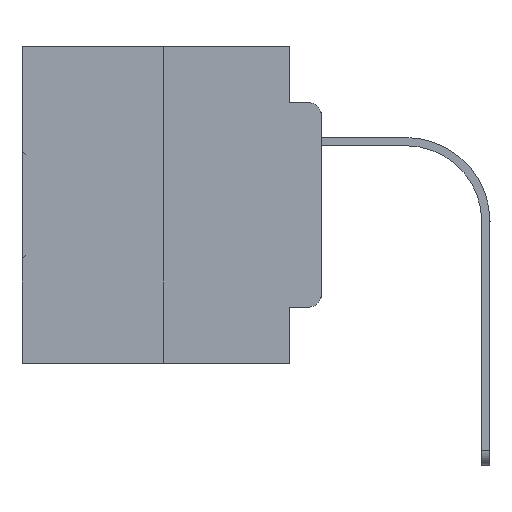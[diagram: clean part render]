
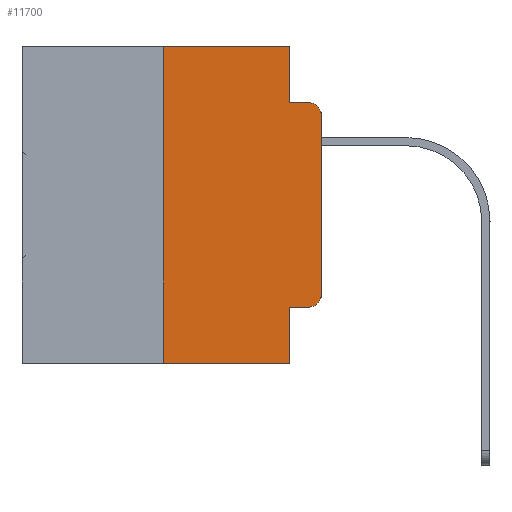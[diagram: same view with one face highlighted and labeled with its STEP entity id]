
A CAD part, left-side view. The second image highlights one B-rep face of the part: STEP entity #11700.
In plain terms, the highlighted planar face has unit normal (-1, 0, 0).
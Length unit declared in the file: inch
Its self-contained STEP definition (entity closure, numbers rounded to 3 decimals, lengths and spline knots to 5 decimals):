
#168 = DIRECTION ( 'NONE',  ( 0., 0., -1. ) ) ;
#213 = VERTEX_POINT ( 'NONE', #25439 ) ;
#641 = CARTESIAN_POINT ( 'NONE',  ( 0., 0.051, -0.5 ) ) ;
#700 = VERTEX_POINT ( 'NONE', #30990 ) ;
#843 = VERTEX_POINT ( 'NONE', #4850 ) ;
#1678 = AXIS2_PLACEMENT_3D ( 'NONE', #29289, #9576, #21879 ) ;
#1745 = DIRECTION ( 'NONE',  ( 0., -1., 0. ) ) ;
#2567 = CARTESIAN_POINT ( 'NONE',  ( 0., 0.473, 0. ) ) ;
#2694 = CIRCLE ( 'NONE', #1678, 0.02 ) ;
#2967 = DIRECTION ( 'NONE',  ( 0., 0., 1. ) ) ;
#3023 = ORIENTED_EDGE ( 'NONE', *, *, #15498, .T. ) ;
#3044 = AXIS2_PLACEMENT_3D ( 'NONE', #2567, #4975, #14767 ) ;
#3327 = CARTESIAN_POINT ( 'NONE',  ( 0., 0.051, 0. ) ) ;
#3491 = CARTESIAN_POINT ( 'NONE',  ( 0., 0.051, 0. ) ) ;
#3603 = CARTESIAN_POINT ( 'NONE',  ( 0., 0.051, -0.4115 ) ) ;
#4026 = DIRECTION ( 'NONE',  ( 0., -1., 0. ) ) ;
#4403 = VECTOR ( 'NONE', #26647, 39.37008 ) ;
#4667 = CARTESIAN_POINT ( 'NONE',  ( 0., 0.473, -0.5 ) ) ;
#4699 = LINE ( 'NONE', #7105, #4403 ) ;
#4794 = LINE ( 'NONE', #7355, #26368 ) ;
#4845 = ORIENTED_EDGE ( 'NONE', *, *, #5979, .F. ) ;
#4850 = CARTESIAN_POINT ( 'NONE',  ( 0., 0., -0.3915 ) ) ;
#4957 = VECTOR ( 'NONE', #4026, 39.37008 ) ;
#4975 = DIRECTION ( 'NONE',  ( 1., 0., 0. ) ) ;
#5979 = EDGE_CURVE ( 'NONE', #22301, #213, #17883, .T. ) ;
#6048 = CARTESIAN_POINT ( 'NONE',  ( 0., 0.051, -0.0885 ) ) ;
#6679 = VECTOR ( 'NONE', #2967, 39.37008 ) ;
#6813 = VECTOR ( 'NONE', #1745, 39.37008 ) ;
#7105 = CARTESIAN_POINT ( 'NONE',  ( 0., 0., 0. ) ) ;
#7355 = CARTESIAN_POINT ( 'NONE',  ( 0., 0.051, -0.4115 ) ) ;
#7389 = PLANE ( 'NONE',  #3044 ) ;
#7409 = EDGE_CURVE ( 'NONE', #13861, #18102, #20926, .T. ) ;
#9336 = ORIENTED_EDGE ( 'NONE', *, *, #7409, .F. ) ;
#9576 = DIRECTION ( 'NONE',  ( -1., 0., 0. ) ) ;
#10498 = EDGE_CURVE ( 'NONE', #19987, #18843, #12810, .T. ) ;
#11436 = CARTESIAN_POINT ( 'NONE',  ( 0., 0.02, -0.3915 ) ) ;
#11700 = ADVANCED_FACE ( 'NONE', ( #20336 ), #7389, .F. ) ;
#12506 = DIRECTION ( 'NONE',  ( 0., -1., 0. ) ) ;
#12810 = LINE ( 'NONE', #6048, #19363 ) ;
#13243 = EDGE_CURVE ( 'NONE', #213, #700, #31411, .T. ) ;
#13283 = DIRECTION ( 'NONE',  ( 0., 0., -1. ) ) ;
#13342 = ORIENTED_EDGE ( 'NONE', *, *, #28454, .T. ) ;
#13861 = VERTEX_POINT ( 'NONE', #3603 ) ;
#14296 = LINE ( 'NONE', #4667, #4957 ) ;
#14767 = DIRECTION ( 'NONE',  ( 0., 0., -1. ) ) ;
#15382 = EDGE_CURVE ( 'NONE', #22301, #18102, #14296, .T. ) ;
#15498 = EDGE_CURVE ( 'NONE', #26483, #843, #31577, .T. ) ;
#15684 = LINE ( 'NONE', #3327, #27920 ) ;
#15959 = CARTESIAN_POINT ( 'NONE',  ( 0., 0.25, -0.5 ) ) ;
#16174 = CARTESIAN_POINT ( 'NONE',  ( 0., 0.02, -0.0885 ) ) ;
#17610 = EDGE_CURVE ( 'NONE', #30897, #18843, #2694, .T. ) ;
#17744 = AXIS2_PLACEMENT_3D ( 'NONE', #11436, #21168, #168 ) ;
#17883 = LINE ( 'NONE', #27662, #6679 ) ;
#18102 = VERTEX_POINT ( 'NONE', #641 ) ;
#18532 = ORIENTED_EDGE ( 'NONE', *, *, #21946, .F. ) ;
#18843 = VERTEX_POINT ( 'NONE', #16174 ) ;
#18986 = ORIENTED_EDGE ( 'NONE', *, *, #21766, .T. ) ;
#19210 = CARTESIAN_POINT ( 'NONE',  ( 0., 0.473, 0. ) ) ;
#19363 = VECTOR ( 'NONE', #30105, 39.37008 ) ;
#19397 = CARTESIAN_POINT ( 'NONE',  ( 0., 0.02, -0.4115 ) ) ;
#19561 = VECTOR ( 'NONE', #13283, 39.37008 ) ;
#19987 = VERTEX_POINT ( 'NONE', #31288 ) ;
#20336 = FACE_OUTER_BOUND ( 'NONE', #30190, .T. ) ;
#20926 = LINE ( 'NONE', #3491, #19561 ) ;
#21168 = DIRECTION ( 'NONE',  ( -1., 0., 0. ) ) ;
#21714 = CARTESIAN_POINT ( 'NONE',  ( 0., 0., -0.1085 ) ) ;
#21766 = EDGE_CURVE ( 'NONE', #13861, #26483, #4794, .T. ) ;
#21879 = DIRECTION ( 'NONE',  ( 0., 0., -1. ) ) ;
#21946 = EDGE_CURVE ( 'NONE', #700, #19987, #15684, .T. ) ;
#22301 = VERTEX_POINT ( 'NONE', #15959 ) ;
#24225 = ORIENTED_EDGE ( 'NONE', *, *, #13243, .F. ) ;
#25439 = CARTESIAN_POINT ( 'NONE',  ( 0., 0.25, 0. ) ) ;
#26252 = ORIENTED_EDGE ( 'NONE', *, *, #15382, .T. ) ;
#26368 = VECTOR ( 'NONE', #12506, 39.37008 ) ;
#26483 = VERTEX_POINT ( 'NONE', #19397 ) ;
#26647 = DIRECTION ( 'NONE',  ( 0., 0., 1. ) ) ;
#27662 = CARTESIAN_POINT ( 'NONE',  ( 0., 0.25, 0. ) ) ;
#27920 = VECTOR ( 'NONE', #30100, 39.37008 ) ;
#28259 = ORIENTED_EDGE ( 'NONE', *, *, #10498, .F. ) ;
#28454 = EDGE_CURVE ( 'NONE', #843, #30897, #4699, .T. ) ;
#29289 = CARTESIAN_POINT ( 'NONE',  ( 0., 0.02, -0.1085 ) ) ;
#30100 = DIRECTION ( 'NONE',  ( 0., 0., -1. ) ) ;
#30105 = DIRECTION ( 'NONE',  ( 0., -1., 0. ) ) ;
#30190 = EDGE_LOOP ( 'NONE', ( #13342, #30502, #28259, #18532, #24225, #4845, #26252, #9336, #18986, #3023 ) ) ;
#30502 = ORIENTED_EDGE ( 'NONE', *, *, #17610, .T. ) ;
#30897 = VERTEX_POINT ( 'NONE', #21714 ) ;
#30990 = CARTESIAN_POINT ( 'NONE',  ( 0., 0.051, 0. ) ) ;
#31288 = CARTESIAN_POINT ( 'NONE',  ( 0., 0.051, -0.0885 ) ) ;
#31411 = LINE ( 'NONE', #19210, #6813 ) ;
#31577 = CIRCLE ( 'NONE', #17744, 0.02 ) ;
